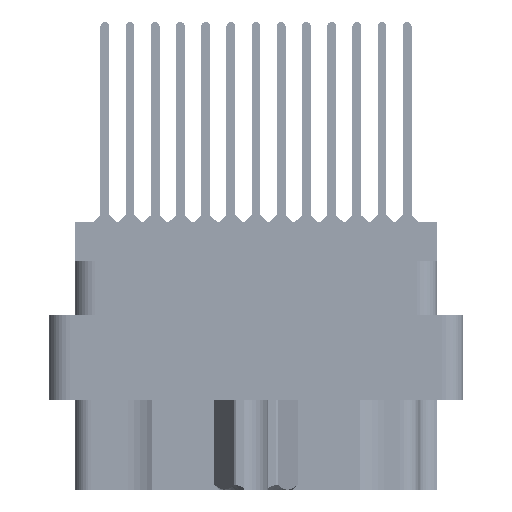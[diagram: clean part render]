
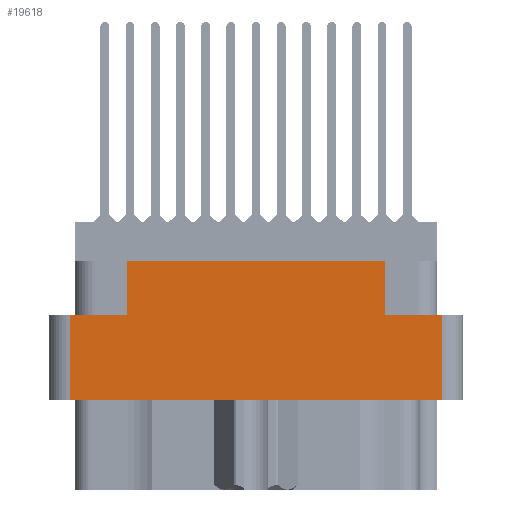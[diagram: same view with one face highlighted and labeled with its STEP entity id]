
A CAD part, left-side view. The second image highlights one B-rep face of the part: STEP entity #19618.
In plain terms, the highlighted planar face has unit normal (-1, 0, 0).
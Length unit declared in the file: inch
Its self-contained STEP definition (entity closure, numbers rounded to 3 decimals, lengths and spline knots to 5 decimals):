
#155 = VERTEX_POINT ( 'NONE', #67985 ) ;
#171 = PLANE ( 'NONE',  #82110 ) ;
#665 = CARTESIAN_POINT ( 'NONE',  ( -1.359, 0.555, -0.798 ) ) ;
#737 = ORIENTED_EDGE ( 'NONE', *, *, #59048, .F. ) ;
#1982 = ORIENTED_EDGE ( 'NONE', *, *, #64321, .F. ) ;
#2816 = VECTOR ( 'NONE', #33367, 39.37008 ) ;
#3407 = CARTESIAN_POINT ( 'NONE',  ( -1.359, -0.555, -0.529 ) ) ;
#4576 = DIRECTION ( 'NONE',  ( 0., 0., 1. ) ) ;
#4911 = LINE ( 'NONE', #35761, #71566 ) ;
#6112 = CARTESIAN_POINT ( 'NONE',  ( -1.359, -0.617, -0.798 ) ) ;
#6201 = EDGE_CURVE ( 'NONE', #8341, #155, #6893, .T. ) ;
#6893 = LINE ( 'NONE', #38986, #55392 ) ;
#6933 = DIRECTION ( 'NONE',  ( 0., 0., 1. ) ) ;
#8341 = VERTEX_POINT ( 'NONE', #3407 ) ;
#9347 = VECTOR ( 'NONE', #4576, 39.37008 ) ;
#11750 = CARTESIAN_POINT ( 'NONE',  ( -1.359, 0.617, -0.117 ) ) ;
#11847 = VERTEX_POINT ( 'NONE', #48031 ) ;
#14884 = ORIENTED_EDGE ( 'NONE', *, *, #18443, .T. ) ;
#18419 = VERTEX_POINT ( 'NONE', #26331 ) ;
#18443 = EDGE_CURVE ( 'NONE', #11847, #155, #44167, .T. ) ;
#19463 = VERTEX_POINT ( 'NONE', #50438 ) ;
#19604 = DIRECTION ( 'NONE',  ( -1., 0., 0. ) ) ;
#19618 = ADVANCED_FACE ( 'NONE', ( #68275 ), #171, .T. ) ;
#20814 = LINE ( 'NONE', #25859, #43008 ) ;
#21008 = CARTESIAN_POINT ( 'NONE',  ( -1.359, 0.3825, -0.277 ) ) ;
#25816 = ORIENTED_EDGE ( 'NONE', *, *, #52418, .T. ) ;
#25859 = CARTESIAN_POINT ( 'NONE',  ( -1.359, 0., -0.277 ) ) ;
#26331 = CARTESIAN_POINT ( 'NONE',  ( -1.359, 0.3825, -0.117 ) ) ;
#28295 = VECTOR ( 'NONE', #73665, 39.37008 ) ;
#30481 = CARTESIAN_POINT ( 'NONE',  ( -1.359, -0.555, -0.277 ) ) ;
#31787 = DIRECTION ( 'NONE',  ( 0., -1., 0. ) ) ;
#33367 = DIRECTION ( 'NONE',  ( 0., 0., -1. ) ) ;
#33974 = DIRECTION ( 'NONE',  ( 0., 0., 1. ) ) ;
#34394 = CARTESIAN_POINT ( 'NONE',  ( -1.359, -0.555, -0.798 ) ) ;
#34660 = ORIENTED_EDGE ( 'NONE', *, *, #68358, .F. ) ;
#34944 = VERTEX_POINT ( 'NONE', #53181 ) ;
#35761 = CARTESIAN_POINT ( 'NONE',  ( -1.359, 0., -0.277 ) ) ;
#38233 = DIRECTION ( 'NONE',  ( 0., -1., 0. ) ) ;
#38530 = VECTOR ( 'NONE', #38233, 39.37008 ) ;
#38986 = CARTESIAN_POINT ( 'NONE',  ( -1.359, 0., -0.529 ) ) ;
#40871 = EDGE_CURVE ( 'NONE', #69139, #34944, #71977, .T. ) ;
#43008 = VECTOR ( 'NONE', #31787, 39.37008 ) ;
#44167 = LINE ( 'NONE', #665, #2816 ) ;
#44549 = VECTOR ( 'NONE', #33974, 39.37008 ) ;
#48031 = CARTESIAN_POINT ( 'NONE',  ( -1.359, 0.555, -0.277 ) ) ;
#50438 = CARTESIAN_POINT ( 'NONE',  ( -1.359, 0.3825, -0.277 ) ) ;
#52418 = EDGE_CURVE ( 'NONE', #8341, #74763, #75777, .T. ) ;
#53181 = CARTESIAN_POINT ( 'NONE',  ( -1.359, -0.3825, -0.117 ) ) ;
#55392 = VECTOR ( 'NONE', #76858, 39.37008 ) ;
#56180 = CARTESIAN_POINT ( 'NONE',  ( -1.359, -0.3825, -0.277 ) ) ;
#57743 = LINE ( 'NONE', #11750, #38530 ) ;
#57798 = CARTESIAN_POINT ( 'NONE',  ( -1.359, -0.3825, -0.277 ) ) ;
#59048 = EDGE_CURVE ( 'NONE', #18419, #34944, #57743, .T. ) ;
#59349 = ORIENTED_EDGE ( 'NONE', *, *, #40871, .T. ) ;
#63399 = ORIENTED_EDGE ( 'NONE', *, *, #77879, .F. ) ;
#64321 = EDGE_CURVE ( 'NONE', #69139, #74763, #20814, .T. ) ;
#66388 = EDGE_LOOP ( 'NONE', ( #63399, #14884, #71528, #25816, #1982, #59349, #737, #34660 ) ) ;
#67985 = CARTESIAN_POINT ( 'NONE',  ( -1.359, 0.555, -0.529 ) ) ;
#68275 = FACE_OUTER_BOUND ( 'NONE', #66388, .T. ) ;
#68358 = EDGE_CURVE ( 'NONE', #19463, #18419, #70829, .T. ) ;
#69139 = VERTEX_POINT ( 'NONE', #57798 ) ;
#70829 = LINE ( 'NONE', #21008, #44549 ) ;
#71528 = ORIENTED_EDGE ( 'NONE', *, *, #6201, .F. ) ;
#71566 = VECTOR ( 'NONE', #75315, 39.37008 ) ;
#71977 = LINE ( 'NONE', #56180, #9347 ) ;
#73665 = DIRECTION ( 'NONE',  ( 0., 0., 1. ) ) ;
#74763 = VERTEX_POINT ( 'NONE', #30481 ) ;
#75315 = DIRECTION ( 'NONE',  ( 0., -1., 0. ) ) ;
#75777 = LINE ( 'NONE', #34394, #28295 ) ;
#76858 = DIRECTION ( 'NONE',  ( 0., 1., 0. ) ) ;
#77879 = EDGE_CURVE ( 'NONE', #11847, #19463, #4911, .T. ) ;
#82110 = AXIS2_PLACEMENT_3D ( 'NONE', #6112, #19604, #6933 ) ;
